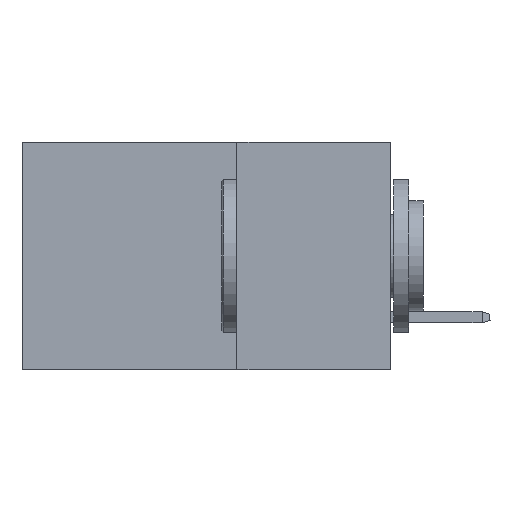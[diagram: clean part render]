
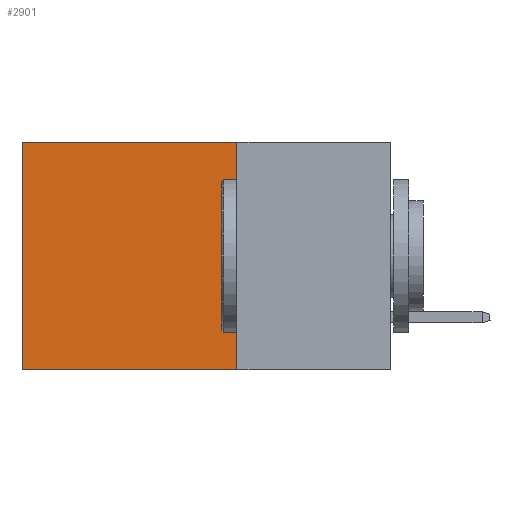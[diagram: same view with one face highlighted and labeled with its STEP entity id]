
A CAD part, left-side view. The second image highlights one B-rep face of the part: STEP entity #2901.
In plain terms, the highlighted planar face has unit normal (-1, 0, 0).
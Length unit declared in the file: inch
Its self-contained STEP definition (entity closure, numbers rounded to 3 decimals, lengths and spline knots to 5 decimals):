
#151 = EDGE_CURVE ( 'NONE', #24123, #7072, #5110, .T. ) ;
#1048 = CARTESIAN_POINT ( 'NONE',  ( 0.2875, 0.25, 0. ) ) ;
#1756 = CARTESIAN_POINT ( 'NONE',  ( 0.2875, 0.25, -0.37 ) ) ;
#2300 = DIRECTION ( 'NONE',  ( 1., 0., 0. ) ) ;
#2901 = ADVANCED_FACE ( 'NONE', ( #16044 ), #15239, .F. ) ;
#5110 = LINE ( 'NONE', #21987, #9860 ) ;
#6555 = ORIENTED_EDGE ( 'NONE', *, *, #11408, .T. ) ;
#7072 = VERTEX_POINT ( 'NONE', #8209 ) ;
#7592 = DIRECTION ( 'NONE',  ( 0., 1., 0. ) ) ;
#7867 = LINE ( 'NONE', #1048, #21386 ) ;
#8209 = CARTESIAN_POINT ( 'NONE',  ( 0.2875, 0.25, -0.37 ) ) ;
#8613 = EDGE_LOOP ( 'NONE', ( #6555, #18510, #22136, #15705 ) ) ;
#9282 = CARTESIAN_POINT ( 'NONE',  ( 0.2875, 0.6, -0.37 ) ) ;
#9638 = LINE ( 'NONE', #24443, #13659 ) ;
#9860 = VECTOR ( 'NONE', #17354, 39.37008 ) ;
#10554 = AXIS2_PLACEMENT_3D ( 'NONE', #19585, #2300, #27967 ) ;
#11223 = EDGE_CURVE ( 'NONE', #7072, #23413, #16393, .T. ) ;
#11238 = DIRECTION ( 'NONE',  ( 0., 1., 0. ) ) ;
#11408 = EDGE_CURVE ( 'NONE', #25141, #23413, #9638, .T. ) ;
#12070 = EDGE_CURVE ( 'NONE', #24123, #25141, #7867, .T. ) ;
#13659 = VECTOR ( 'NONE', #26705, 39.37008 ) ;
#15239 = PLANE ( 'NONE',  #10554 ) ;
#15705 = ORIENTED_EDGE ( 'NONE', *, *, #12070, .T. ) ;
#16044 = FACE_OUTER_BOUND ( 'NONE', #8613, .T. ) ;
#16393 = LINE ( 'NONE', #1756, #19057 ) ;
#16884 = CARTESIAN_POINT ( 'NONE',  ( 0.2875, 0.6, 0. ) ) ;
#16953 = CARTESIAN_POINT ( 'NONE',  ( 0.2875, 0.25, 0. ) ) ;
#17354 = DIRECTION ( 'NONE',  ( 0., 0., -1. ) ) ;
#18510 = ORIENTED_EDGE ( 'NONE', *, *, #11223, .F. ) ;
#19057 = VECTOR ( 'NONE', #11238, 39.37008 ) ;
#19585 = CARTESIAN_POINT ( 'NONE',  ( 0.2875, 0.25, 0. ) ) ;
#21386 = VECTOR ( 'NONE', #7592, 39.37008 ) ;
#21987 = CARTESIAN_POINT ( 'NONE',  ( 0.2875, 0.25, 0. ) ) ;
#22136 = ORIENTED_EDGE ( 'NONE', *, *, #151, .F. ) ;
#23413 = VERTEX_POINT ( 'NONE', #9282 ) ;
#24123 = VERTEX_POINT ( 'NONE', #16953 ) ;
#24443 = CARTESIAN_POINT ( 'NONE',  ( 0.2875, 0.6, 0. ) ) ;
#25141 = VERTEX_POINT ( 'NONE', #16884 ) ;
#26705 = DIRECTION ( 'NONE',  ( 0., 0., -1. ) ) ;
#27967 = DIRECTION ( 'NONE',  ( 0., 0., -1. ) ) ;
